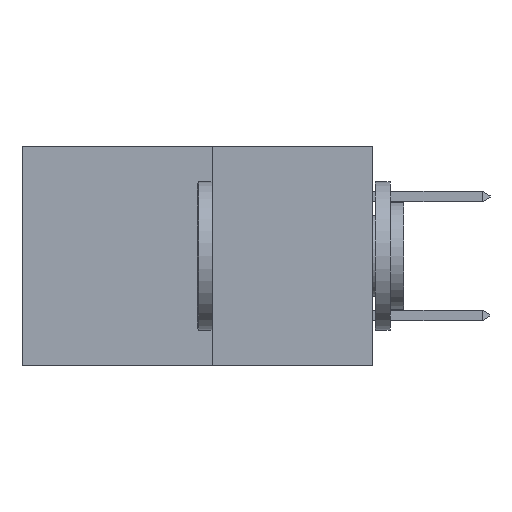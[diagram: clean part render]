
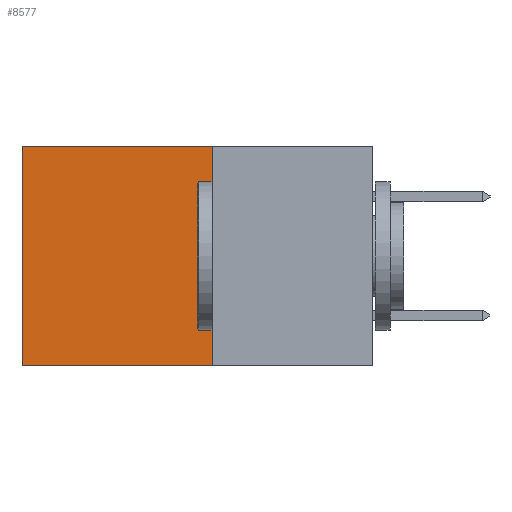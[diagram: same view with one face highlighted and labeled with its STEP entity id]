
A CAD part, left-side view. The second image highlights one B-rep face of the part: STEP entity #8577.
In plain terms, the highlighted planar face has unit normal (-1, 0, 0).
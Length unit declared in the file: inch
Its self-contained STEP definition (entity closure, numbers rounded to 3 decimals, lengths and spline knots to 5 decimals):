
#448 = CARTESIAN_POINT ( 'NONE',  ( 0.277, 0.59, -0.37 ) ) ;
#1205 = ORIENTED_EDGE ( 'NONE', *, *, #6289, .T. ) ;
#1504 = EDGE_CURVE ( 'NONE', #17287, #15101, #10117, .T. ) ;
#1885 = DIRECTION ( 'NONE',  ( 0., 0., -1. ) ) ;
#2828 = VECTOR ( 'NONE', #12102, 39.37008 ) ;
#3579 = EDGE_CURVE ( 'NONE', #5393, #15101, #11345, .T. ) ;
#4172 = VECTOR ( 'NONE', #10376, 39.37008 ) ;
#4658 = CARTESIAN_POINT ( 'NONE',  ( 0.277, 0.59, -0.37 ) ) ;
#4991 = DIRECTION ( 'NONE',  ( 0., 0., -1. ) ) ;
#5393 = VERTEX_POINT ( 'NONE', #15658 ) ;
#6289 = EDGE_CURVE ( 'NONE', #15863, #17287, #10105, .T. ) ;
#6495 = VECTOR ( 'NONE', #6788, 39.37008 ) ;
#6788 = DIRECTION ( 'NONE',  ( 0., 1., 0. ) ) ;
#6848 = CARTESIAN_POINT ( 'NONE',  ( 0.277, 0.27, 0. ) ) ;
#6939 = VECTOR ( 'NONE', #1885, 39.37008 ) ;
#7203 = ORIENTED_EDGE ( 'NONE', *, *, #1504, .T. ) ;
#7645 = CARTESIAN_POINT ( 'NONE',  ( 0.277, 0.27, -0.37 ) ) ;
#8355 = ORIENTED_EDGE ( 'NONE', *, *, #3579, .F. ) ;
#8577 = ADVANCED_FACE ( 'NONE', ( #10439 ), #11708, .F. ) ;
#9379 = CARTESIAN_POINT ( 'NONE',  ( 0.277, 0.27, -0.37 ) ) ;
#9515 = EDGE_CURVE ( 'NONE', #15863, #5393, #9982, .T. ) ;
#9982 = LINE ( 'NONE', #13459, #2828 ) ;
#10105 = LINE ( 'NONE', #6848, #6495 ) ;
#10117 = LINE ( 'NONE', #4658, #6939 ) ;
#10376 = DIRECTION ( 'NONE',  ( 0., 1., 0. ) ) ;
#10404 = AXIS2_PLACEMENT_3D ( 'NONE', #7645, #13081, #4991 ) ;
#10439 = FACE_OUTER_BOUND ( 'NONE', #10786, .T. ) ;
#10786 = EDGE_LOOP ( 'NONE', ( #7203, #8355, #11288, #1205 ) ) ;
#11288 = ORIENTED_EDGE ( 'NONE', *, *, #9515, .F. ) ;
#11345 = LINE ( 'NONE', #9379, #4172 ) ;
#11708 = PLANE ( 'NONE',  #10404 ) ;
#12102 = DIRECTION ( 'NONE',  ( 0., 0., -1. ) ) ;
#13081 = DIRECTION ( 'NONE',  ( 1., 0., 0. ) ) ;
#13459 = CARTESIAN_POINT ( 'NONE',  ( 0.277, 0.27, -0.37 ) ) ;
#14046 = CARTESIAN_POINT ( 'NONE',  ( 0.277, 0.27, 0. ) ) ;
#15101 = VERTEX_POINT ( 'NONE', #448 ) ;
#15658 = CARTESIAN_POINT ( 'NONE',  ( 0.277, 0.27, -0.37 ) ) ;
#15863 = VERTEX_POINT ( 'NONE', #14046 ) ;
#16625 = CARTESIAN_POINT ( 'NONE',  ( 0.277, 0.59, 0. ) ) ;
#17287 = VERTEX_POINT ( 'NONE', #16625 ) ;
